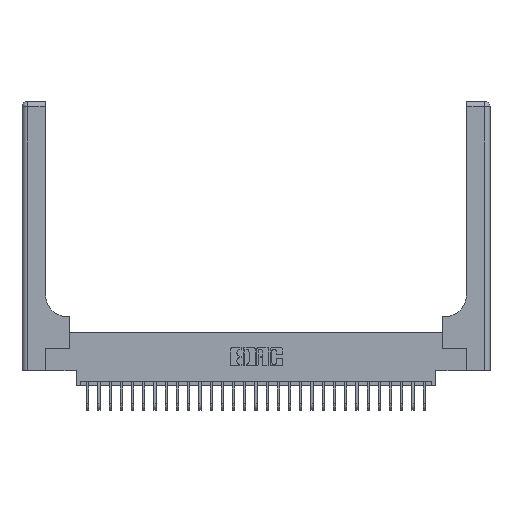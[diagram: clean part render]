
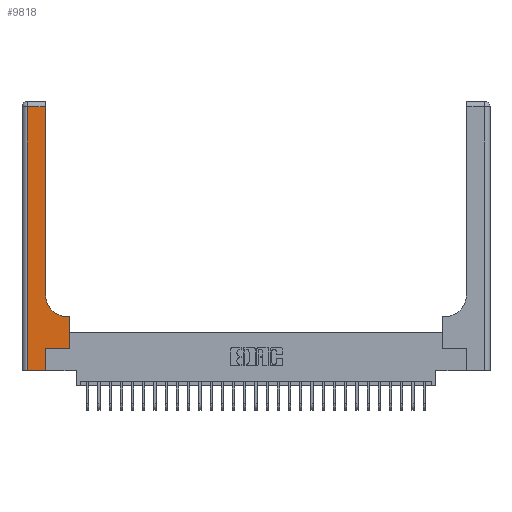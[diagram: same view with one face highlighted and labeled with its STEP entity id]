
A CAD part, top view. The second image highlights one B-rep face of the part: STEP entity #9818.
In plain terms, the highlighted planar face has unit normal (0, 0, 1).
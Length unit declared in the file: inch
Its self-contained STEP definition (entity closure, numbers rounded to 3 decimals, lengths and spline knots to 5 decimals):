
#998 = CARTESIAN_POINT ( 'NONE',  ( 0., 3., 0.37 ) ) ;
#1301 = AXIS2_PLACEMENT_3D ( 'NONE', #998, #16480, #21110 ) ;
#1376 = ORIENTED_EDGE ( 'NONE', *, *, #18785, .T. ) ;
#1450 = CARTESIAN_POINT ( 'NONE',  ( 0.26, 0.85, 0.37 ) ) ;
#1608 = VECTOR ( 'NONE', #2937, 39.37008 ) ;
#1965 = DIRECTION ( 'NONE',  ( 0., 1., 0. ) ) ;
#2121 = VECTOR ( 'NONE', #8770, 39.37008 ) ;
#2233 = ORIENTED_EDGE ( 'NONE', *, *, #12861, .T. ) ;
#2445 = CARTESIAN_POINT ( 'NONE',  ( 0.26, 3., 0.37 ) ) ;
#2503 = CARTESIAN_POINT ( 'NONE',  ( 0.06, 0., 0.37 ) ) ;
#2612 = CARTESIAN_POINT ( 'NONE',  ( 0., 2.94, 0.37 ) ) ;
#2935 = LINE ( 'NONE', #2612, #3295 ) ;
#2937 = DIRECTION ( 'NONE',  ( 0., -1., 0. ) ) ;
#3295 = VECTOR ( 'NONE', #11548, 39.37008 ) ;
#3958 = VERTEX_POINT ( 'NONE', #26314 ) ;
#4500 = VERTEX_POINT ( 'NONE', #1450 ) ;
#4970 = VERTEX_POINT ( 'NONE', #25996 ) ;
#5373 = VERTEX_POINT ( 'NONE', #10507 ) ;
#5473 = ORIENTED_EDGE ( 'NONE', *, *, #13938, .T. ) ;
#5635 = LINE ( 'NONE', #6381, #7017 ) ;
#5639 = ORIENTED_EDGE ( 'NONE', *, *, #6017, .T. ) ;
#6002 = DIRECTION ( 'NONE',  ( 0., 1., 0. ) ) ;
#6017 = EDGE_CURVE ( 'NONE', #20009, #10663, #2935, .T. ) ;
#6381 = CARTESIAN_POINT ( 'NONE',  ( 0.26, 0.6, 0.37 ) ) ;
#6443 = DIRECTION ( 'NONE',  ( 1., 0., 0. ) ) ;
#7017 = VECTOR ( 'NONE', #22338, 39.37008 ) ;
#7111 = DIRECTION ( 'NONE',  ( 0., 1., 0. ) ) ;
#7577 = FACE_OUTER_BOUND ( 'NONE', #8387, .T. ) ;
#8387 = EDGE_LOOP ( 'NONE', ( #1376, #5639, #14386, #9006, #10328, #22079, #5473, #26401, #2233 ) ) ;
#8770 = DIRECTION ( 'NONE',  ( 1., 0., 0. ) ) ;
#9006 = ORIENTED_EDGE ( 'NONE', *, *, #10329, .T. ) ;
#9462 = CARTESIAN_POINT ( 'NONE',  ( 0.528, 0.6, 0.37 ) ) ;
#9722 = LINE ( 'NONE', #21977, #2121 ) ;
#9818 = ADVANCED_FACE ( 'NONE', ( #7577 ), #9823, .F. ) ;
#9823 = PLANE ( 'NONE',  #1301 ) ;
#10141 = LINE ( 'NONE', #21803, #11896 ) ;
#10328 = ORIENTED_EDGE ( 'NONE', *, *, #21990, .T. ) ;
#10329 = EDGE_CURVE ( 'NONE', #15975, #4970, #16553, .T. ) ;
#10507 = CARTESIAN_POINT ( 'NONE',  ( 0.528, 0.25, 0.37 ) ) ;
#10663 = VERTEX_POINT ( 'NONE', #12994 ) ;
#10955 = DIRECTION ( 'NONE',  ( 0., 0., -1. ) ) ;
#11152 = CARTESIAN_POINT ( 'NONE',  ( 0.51, 0.85, 0.37 ) ) ;
#11376 = VECTOR ( 'NONE', #6443, 39.37008 ) ;
#11548 = DIRECTION ( 'NONE',  ( -1., 0., 0. ) ) ;
#11562 = EDGE_CURVE ( 'NONE', #10663, #15975, #15490, .T. ) ;
#11794 = CARTESIAN_POINT ( 'NONE',  ( 0.26, 2.94, 0.37 ) ) ;
#11896 = VECTOR ( 'NONE', #1965, 39.37008 ) ;
#12861 = EDGE_CURVE ( 'NONE', #3958, #4500, #13361, .T. ) ;
#12994 = CARTESIAN_POINT ( 'NONE',  ( 0.06, 2.94, 0.37 ) ) ;
#13074 = CARTESIAN_POINT ( 'NONE',  ( 0.265, 0.25, 0.37 ) ) ;
#13148 = VECTOR ( 'NONE', #7111, 39.37008 ) ;
#13361 = CIRCLE ( 'NONE', #22624, 0.25 ) ;
#13938 = EDGE_CURVE ( 'NONE', #5373, #21594, #22020, .T. ) ;
#14386 = ORIENTED_EDGE ( 'NONE', *, *, #11562, .T. ) ;
#15490 = LINE ( 'NONE', #25197, #1608 ) ;
#15605 = DIRECTION ( 'NONE',  ( 1., 0., 0. ) ) ;
#15975 = VERTEX_POINT ( 'NONE', #2503 ) ;
#16258 = VERTEX_POINT ( 'NONE', #13074 ) ;
#16480 = DIRECTION ( 'NONE',  ( 0., 0., -1. ) ) ;
#16509 = CARTESIAN_POINT ( 'NONE',  ( 0.528, 0.25, 0.37 ) ) ;
#16553 = LINE ( 'NONE', #24158, #11376 ) ;
#16602 = EDGE_CURVE ( 'NONE', #21594, #3958, #5635, .T. ) ;
#17169 = EDGE_CURVE ( 'NONE', #16258, #5373, #9722, .T. ) ;
#18785 = EDGE_CURVE ( 'NONE', #4500, #20009, #28110, .T. ) ;
#18807 = VECTOR ( 'NONE', #6002, 39.37008 ) ;
#20009 = VERTEX_POINT ( 'NONE', #11794 ) ;
#21110 = DIRECTION ( 'NONE',  ( -1., 0., 0. ) ) ;
#21594 = VERTEX_POINT ( 'NONE', #9462 ) ;
#21803 = CARTESIAN_POINT ( 'NONE',  ( 0.265, 0., 0.37 ) ) ;
#21977 = CARTESIAN_POINT ( 'NONE',  ( 0.265, 0.25, 0.37 ) ) ;
#21990 = EDGE_CURVE ( 'NONE', #4970, #16258, #10141, .T. ) ;
#22020 = LINE ( 'NONE', #16509, #18807 ) ;
#22079 = ORIENTED_EDGE ( 'NONE', *, *, #17169, .T. ) ;
#22338 = DIRECTION ( 'NONE',  ( -1., 0., 0. ) ) ;
#22624 = AXIS2_PLACEMENT_3D ( 'NONE', #11152, #10955, #15605 ) ;
#24158 = CARTESIAN_POINT ( 'NONE',  ( 0., 0., 0.37 ) ) ;
#25197 = CARTESIAN_POINT ( 'NONE',  ( 0.06, 3., 0.37 ) ) ;
#25996 = CARTESIAN_POINT ( 'NONE',  ( 0.265, 0., 0.37 ) ) ;
#26314 = CARTESIAN_POINT ( 'NONE',  ( 0.51, 0.6, 0.37 ) ) ;
#26401 = ORIENTED_EDGE ( 'NONE', *, *, #16602, .T. ) ;
#28110 = LINE ( 'NONE', #2445, #13148 ) ;
